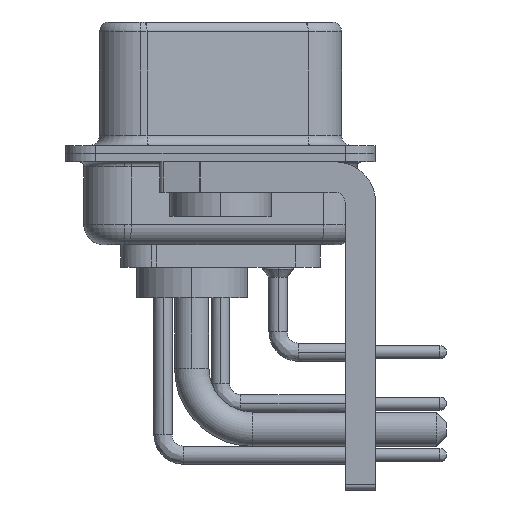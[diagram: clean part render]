
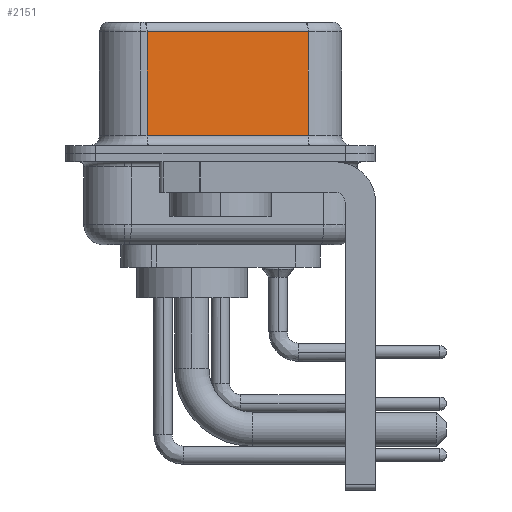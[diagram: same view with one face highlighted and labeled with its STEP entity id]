
A CAD part, left-side view. The second image highlights one B-rep face of the part: STEP entity #2151.
In plain terms, the highlighted planar face has unit normal (-0.985, -0.174, 0).
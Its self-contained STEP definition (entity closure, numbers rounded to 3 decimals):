
#516 = VECTOR ( 'NONE', #21191, 1000. ) ;
#896 = VERTEX_POINT ( 'NONE', #24383 ) ;
#1047 = VECTOR ( 'NONE', #18282, 1000. ) ;
#2151 = ADVANCED_FACE ( 'NONE', ( #18680 ), #24338, .F. ) ;
#2485 = EDGE_CURVE ( 'NONE', #34737, #8951, #17937, .T. ) ;
#3343 = CARTESIAN_POINT ( 'NONE',  ( 3.73, 3.628, 6.52 ) ) ;
#5139 = DIRECTION ( 'NONE',  ( 0.985, 0.174, 0. ) ) ;
#6678 = LINE ( 'NONE', #17521, #13602 ) ;
#7069 = CARTESIAN_POINT ( 'NONE',  ( 5.132, -4.322, 6.02 ) ) ;
#7500 = CARTESIAN_POINT ( 'NONE',  ( 5.132, -4.322, 0.9 ) ) ;
#8538 = LINE ( 'NONE', #3343, #22628 ) ;
#8951 = VERTEX_POINT ( 'NONE', #28165 ) ;
#10483 = CARTESIAN_POINT ( 'NONE',  ( 5.132, -4.322, 6.52 ) ) ;
#11738 = EDGE_CURVE ( 'NONE', #21752, #896, #31856, .T. ) ;
#13220 = EDGE_LOOP ( 'NONE', ( #19079, #33639, #34455, #25112 ) ) ;
#13514 = EDGE_CURVE ( 'NONE', #34737, #896, #6678, .T. ) ;
#13602 = VECTOR ( 'NONE', #35166, 1000. ) ;
#16522 = DIRECTION ( 'NONE',  ( -0.174, 0.985, 0. ) ) ;
#17521 = CARTESIAN_POINT ( 'NONE',  ( 5.132, -4.322, 6.52 ) ) ;
#17937 = LINE ( 'NONE', #20249, #1047 ) ;
#18282 = DIRECTION ( 'NONE',  ( -0.174, 0.985, 0. ) ) ;
#18680 = FACE_OUTER_BOUND ( 'NONE', #13220, .T. ) ;
#19079 = ORIENTED_EDGE ( 'NONE', *, *, #13514, .F. ) ;
#19930 = EDGE_CURVE ( 'NONE', #8951, #21752, #8538, .T. ) ;
#20249 = CARTESIAN_POINT ( 'NONE',  ( 5.132, -4.322, 6.02 ) ) ;
#21191 = DIRECTION ( 'NONE',  ( 0.174, -0.985, 0. ) ) ;
#21752 = VERTEX_POINT ( 'NONE', #21759 ) ;
#21759 = CARTESIAN_POINT ( 'NONE',  ( 3.73, 3.628, 0.9 ) ) ;
#22628 = VECTOR ( 'NONE', #32534, 1000. ) ;
#24338 = PLANE ( 'NONE',  #33293 ) ;
#24383 = CARTESIAN_POINT ( 'NONE',  ( 5.132, -4.322, 0.9 ) ) ;
#25112 = ORIENTED_EDGE ( 'NONE', *, *, #11738, .T. ) ;
#28165 = CARTESIAN_POINT ( 'NONE',  ( 3.73, 3.628, 6.02 ) ) ;
#31856 = LINE ( 'NONE', #7500, #516 ) ;
#32534 = DIRECTION ( 'NONE',  ( 0., 0., -1. ) ) ;
#33293 = AXIS2_PLACEMENT_3D ( 'NONE', #10483, #5139, #16522 ) ;
#33639 = ORIENTED_EDGE ( 'NONE', *, *, #2485, .T. ) ;
#34455 = ORIENTED_EDGE ( 'NONE', *, *, #19930, .T. ) ;
#34737 = VERTEX_POINT ( 'NONE', #7069 ) ;
#35166 = DIRECTION ( 'NONE',  ( 0., 0., -1. ) ) ;
